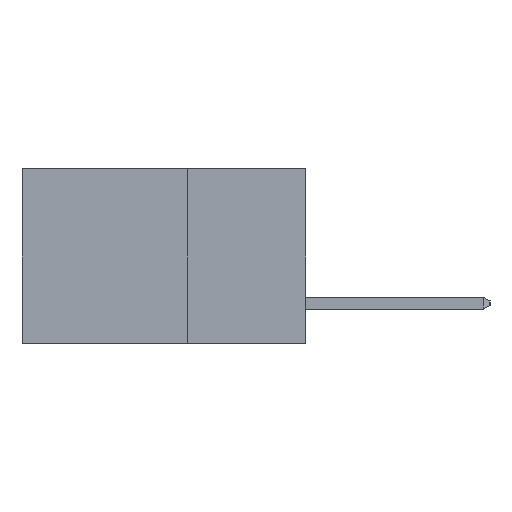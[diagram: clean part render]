
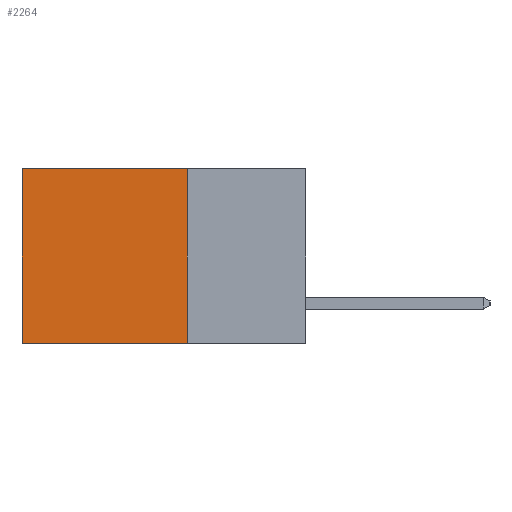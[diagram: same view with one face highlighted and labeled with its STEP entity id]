
A CAD part, left-side view. The second image highlights one B-rep face of the part: STEP entity #2264.
In plain terms, the highlighted planar face has unit normal (-1, 0, 0).
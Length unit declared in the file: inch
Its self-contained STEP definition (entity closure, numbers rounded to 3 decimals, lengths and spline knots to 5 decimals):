
#5 = LINE ( 'NONE', #13712, #12154 ) ;
#54 = VERTEX_POINT ( 'NONE', #10730 ) ;
#560 = VERTEX_POINT ( 'NONE', #4836 ) ;
#1417 = VECTOR ( 'NONE', #14294, 39.37008 ) ;
#1958 = DIRECTION ( 'NONE',  ( 0., 1., 0. ) ) ;
#2264 = ADVANCED_FACE ( 'NONE', ( #15177 ), #2463, .F. ) ;
#2463 = PLANE ( 'NONE',  #13113 ) ;
#2581 = CARTESIAN_POINT ( 'NONE',  ( 0.2615, 0.25, -0.37 ) ) ;
#2958 = ORIENTED_EDGE ( 'NONE', *, *, #13414, .T. ) ;
#3604 = CARTESIAN_POINT ( 'NONE',  ( 0.2615, 0.25, 0. ) ) ;
#4836 = CARTESIAN_POINT ( 'NONE',  ( 0.2615, 0.25, -0.37 ) ) ;
#4860 = VERTEX_POINT ( 'NONE', #13540 ) ;
#5604 = CARTESIAN_POINT ( 'NONE',  ( 0.2615, 0.6, -0.37 ) ) ;
#6138 = DIRECTION ( 'NONE',  ( 0., 0., -1. ) ) ;
#6219 = DIRECTION ( 'NONE',  ( 1., 0., 0. ) ) ;
#6470 = EDGE_CURVE ( 'NONE', #560, #15626, #9842, .T. ) ;
#8345 = CARTESIAN_POINT ( 'NONE',  ( 0.2615, 0.6, -0.37 ) ) ;
#9104 = ORIENTED_EDGE ( 'NONE', *, *, #9236, .F. ) ;
#9236 = EDGE_CURVE ( 'NONE', #54, #560, #5, .T. ) ;
#9842 = LINE ( 'NONE', #14180, #1417 ) ;
#10394 = VECTOR ( 'NONE', #1958, 39.37008 ) ;
#10730 = CARTESIAN_POINT ( 'NONE',  ( 0.2615, 0.25, 0. ) ) ;
#11165 = EDGE_CURVE ( 'NONE', #4860, #15626, #16482, .T. ) ;
#11720 = ORIENTED_EDGE ( 'NONE', *, *, #6470, .F. ) ;
#12154 = VECTOR ( 'NONE', #15255, 39.37008 ) ;
#12317 = VECTOR ( 'NONE', #15108, 39.37008 ) ;
#13113 = AXIS2_PLACEMENT_3D ( 'NONE', #2581, #6219, #6138 ) ;
#13414 = EDGE_CURVE ( 'NONE', #54, #4860, #14623, .T. ) ;
#13540 = CARTESIAN_POINT ( 'NONE',  ( 0.2615, 0.6, 0. ) ) ;
#13712 = CARTESIAN_POINT ( 'NONE',  ( 0.2615, 0.25, -0.37 ) ) ;
#14180 = CARTESIAN_POINT ( 'NONE',  ( 0.2615, 0.25, -0.37 ) ) ;
#14294 = DIRECTION ( 'NONE',  ( 0., 1., 0. ) ) ;
#14556 = ORIENTED_EDGE ( 'NONE', *, *, #11165, .T. ) ;
#14623 = LINE ( 'NONE', #3604, #10394 ) ;
#15108 = DIRECTION ( 'NONE',  ( 0., 0., -1. ) ) ;
#15177 = FACE_OUTER_BOUND ( 'NONE', #19020, .T. ) ;
#15255 = DIRECTION ( 'NONE',  ( 0., 0., -1. ) ) ;
#15626 = VERTEX_POINT ( 'NONE', #8345 ) ;
#16482 = LINE ( 'NONE', #5604, #12317 ) ;
#19020 = EDGE_LOOP ( 'NONE', ( #14556, #11720, #9104, #2958 ) ) ;
